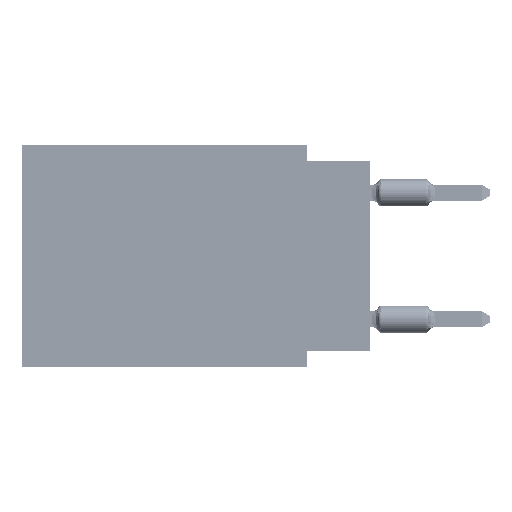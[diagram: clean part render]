
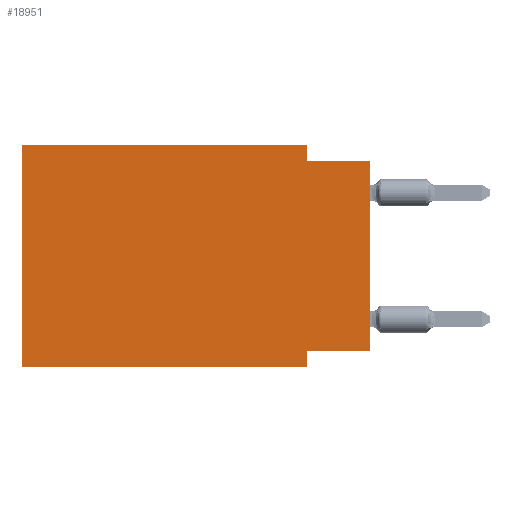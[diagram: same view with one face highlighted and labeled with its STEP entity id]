
A CAD part, left-side view. The second image highlights one B-rep face of the part: STEP entity #18951.
In plain terms, the highlighted planar face has unit normal (-1, 0, 0).
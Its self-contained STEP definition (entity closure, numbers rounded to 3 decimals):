
#2569 = ORIENTED_EDGE ( 'NONE', *, *, #45461, .F. ) ;
#8708 = VERTEX_POINT ( 'NONE', #88572 ) ;
#9171 = DIRECTION ( 'NONE',  ( 0., 0., -1. ) ) ;
#9625 = DIRECTION ( 'NONE',  ( 0., 1., 0. ) ) ;
#11055 = ORIENTED_EDGE ( 'NONE', *, *, #87841, .F. ) ;
#15570 = DIRECTION ( 'NONE',  ( 0., -1., 0. ) ) ;
#15623 = VERTEX_POINT ( 'NONE', #97941 ) ;
#18951 = ADVANCED_FACE ( 'NONE', ( #21441 ), #86108, .F. ) ;
#19022 = CARTESIAN_POINT ( 'NONE',  ( 0., 13.97, 0. ) ) ;
#21287 = CARTESIAN_POINT ( 'NONE',  ( 0., 0., -8.255 ) ) ;
#21441 = FACE_OUTER_BOUND ( 'NONE', #33925, .T. ) ;
#22364 = ORIENTED_EDGE ( 'NONE', *, *, #77136, .F. ) ;
#24841 = EDGE_CURVE ( 'NONE', #116635, #15623, #49047, .T. ) ;
#26628 = LINE ( 'NONE', #64203, #60090 ) ;
#26643 = VECTOR ( 'NONE', #84855, 1000. ) ;
#26785 = VECTOR ( 'NONE', #9625, 1000. ) ;
#27259 = CARTESIAN_POINT ( 'NONE',  ( 0., 0., 0. ) ) ;
#30562 = DIRECTION ( 'NONE',  ( 0., 0., -1. ) ) ;
#32632 = CARTESIAN_POINT ( 'NONE',  ( 0., 2.54, -8.255 ) ) ;
#33925 = EDGE_LOOP ( 'NONE', ( #94938, #2569, #103696, #22364, #11055, #55794, #111687, #64360 ) ) ;
#34819 = CARTESIAN_POINT ( 'NONE',  ( 0., 2.54, 0. ) ) ;
#36546 = CARTESIAN_POINT ( 'NONE',  ( 0., 0., -0.635 ) ) ;
#44325 = VERTEX_POINT ( 'NONE', #85661 ) ;
#45461 = EDGE_CURVE ( 'NONE', #8708, #61330, #103951, .T. ) ;
#47769 = LINE ( 'NONE', #21287, #26785 ) ;
#49047 = LINE ( 'NONE', #86592, #81376 ) ;
#49154 = DIRECTION ( 'NONE',  ( 1., 0., 0. ) ) ;
#49774 = EDGE_CURVE ( 'NONE', #117395, #15623, #118312, .T. ) ;
#50960 = VECTOR ( 'NONE', #69928, 1000. ) ;
#51832 = DIRECTION ( 'NONE',  ( 0., -1., 0. ) ) ;
#52082 = EDGE_CURVE ( 'NONE', #84264, #116635, #47769, .T. ) ;
#52273 = VECTOR ( 'NONE', #51832, 1000. ) ;
#53886 = DIRECTION ( 'NONE',  ( 0., 0., -1. ) ) ;
#55794 = ORIENTED_EDGE ( 'NONE', *, *, #49774, .T. ) ;
#56583 = DIRECTION ( 'NONE',  ( 0., 0., 1. ) ) ;
#60090 = VECTOR ( 'NONE', #15570, 1000. ) ;
#61330 = VERTEX_POINT ( 'NONE', #36546 ) ;
#64203 = CARTESIAN_POINT ( 'NONE',  ( 0., 13.97, 0. ) ) ;
#64360 = ORIENTED_EDGE ( 'NONE', *, *, #52082, .F. ) ;
#69928 = DIRECTION ( 'NONE',  ( 0., 0., 1. ) ) ;
#70543 = LINE ( 'NONE', #27259, #50960 ) ;
#70585 = CARTESIAN_POINT ( 'NONE',  ( 0., 0., -8.255 ) ) ;
#71928 = EDGE_CURVE ( 'NONE', #84264, #61330, #70543, .T. ) ;
#73569 = LINE ( 'NONE', #34819, #87992 ) ;
#74981 = VERTEX_POINT ( 'NONE', #81543 ) ;
#75645 = CARTESIAN_POINT ( 'NONE',  ( 0., 13.97, 0. ) ) ;
#77136 = EDGE_CURVE ( 'NONE', #74981, #44325, #26628, .T. ) ;
#77921 = AXIS2_PLACEMENT_3D ( 'NONE', #75645, #49154, #9171 ) ;
#80767 = CARTESIAN_POINT ( 'NONE',  ( 0., 13.97, -8.89 ) ) ;
#81376 = VECTOR ( 'NONE', #30562, 1000. ) ;
#81543 = CARTESIAN_POINT ( 'NONE',  ( 0., 13.97, 0. ) ) ;
#84264 = VERTEX_POINT ( 'NONE', #70585 ) ;
#84855 = DIRECTION ( 'NONE',  ( 0., -1., 0. ) ) ;
#85661 = CARTESIAN_POINT ( 'NONE',  ( 0., 2.54, 0. ) ) ;
#86108 = PLANE ( 'NONE',  #77921 ) ;
#86592 = CARTESIAN_POINT ( 'NONE',  ( 0., 2.54, -8.89 ) ) ;
#87841 = EDGE_CURVE ( 'NONE', #117395, #74981, #103358, .T. ) ;
#87992 = VECTOR ( 'NONE', #53886, 1000. ) ;
#88572 = CARTESIAN_POINT ( 'NONE',  ( 0., 2.54, -0.635 ) ) ;
#89771 = EDGE_CURVE ( 'NONE', #44325, #8708, #73569, .T. ) ;
#94938 = ORIENTED_EDGE ( 'NONE', *, *, #71928, .T. ) ;
#97941 = CARTESIAN_POINT ( 'NONE',  ( 0., 2.54, -8.89 ) ) ;
#99519 = VECTOR ( 'NONE', #56583, 1000. ) ;
#103358 = LINE ( 'NONE', #19022, #99519 ) ;
#103696 = ORIENTED_EDGE ( 'NONE', *, *, #89771, .F. ) ;
#103951 = LINE ( 'NONE', #104534, #26643 ) ;
#104534 = CARTESIAN_POINT ( 'NONE',  ( 0., 0., -0.635 ) ) ;
#111687 = ORIENTED_EDGE ( 'NONE', *, *, #24841, .F. ) ;
#113654 = CARTESIAN_POINT ( 'NONE',  ( 0., 13.97, -8.89 ) ) ;
#116635 = VERTEX_POINT ( 'NONE', #32632 ) ;
#117395 = VERTEX_POINT ( 'NONE', #113654 ) ;
#118312 = LINE ( 'NONE', #80767, #52273 ) ;
